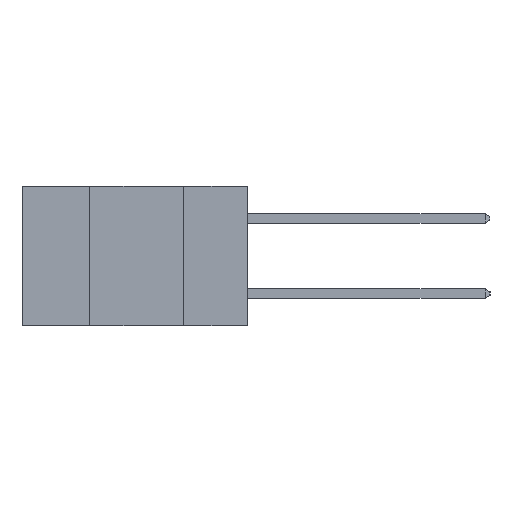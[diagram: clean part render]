
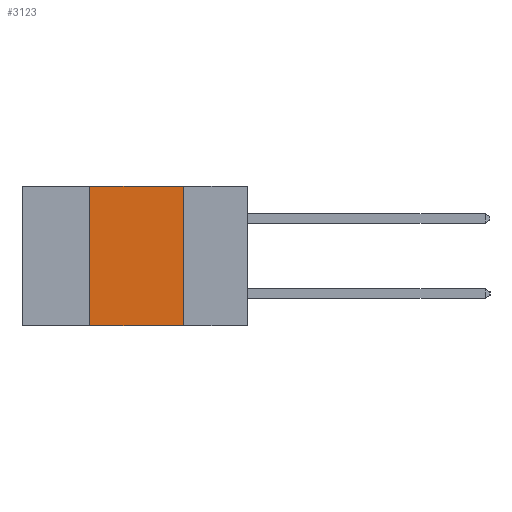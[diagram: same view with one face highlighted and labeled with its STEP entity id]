
A CAD part, left-side view. The second image highlights one B-rep face of the part: STEP entity #3123.
In plain terms, the highlighted planar face has unit normal (-1, 0, 0).
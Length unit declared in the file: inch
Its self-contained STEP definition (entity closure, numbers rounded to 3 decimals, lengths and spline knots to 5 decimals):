
#16 = DIRECTION ( 'NONE',  ( 0., -1., 0. ) ) ;
#35 = CARTESIAN_POINT ( 'NONE',  ( 0., 0.6, 0. ) ) ;
#113 = CARTESIAN_POINT ( 'NONE',  ( 0., 0.42, 0. ) ) ;
#798 = VERTEX_POINT ( 'NONE', #6234 ) ;
#1554 = LINE ( 'NONE', #13496, #13535 ) ;
#2076 = VECTOR ( 'NONE', #3724, 39.37008 ) ;
#3123 = ADVANCED_FACE ( 'NONE', ( #10093 ), #5273, .F. ) ;
#3167 = VERTEX_POINT ( 'NONE', #113 ) ;
#3724 = DIRECTION ( 'NONE',  ( 0., -1., 0. ) ) ;
#3820 = CARTESIAN_POINT ( 'NONE',  ( 0., 0.6, -0.37 ) ) ;
#5273 = PLANE ( 'NONE',  #7773 ) ;
#5826 = LINE ( 'NONE', #35, #14524 ) ;
#6234 = CARTESIAN_POINT ( 'NONE',  ( 0., 0.42, -0.37 ) ) ;
#6297 = VECTOR ( 'NONE', #13851, 39.37008 ) ;
#7108 = VERTEX_POINT ( 'NONE', #8680 ) ;
#7237 = EDGE_CURVE ( 'NONE', #798, #8459, #14017, .T. ) ;
#7324 = ORIENTED_EDGE ( 'NONE', *, *, #7237, .T. ) ;
#7567 = ORIENTED_EDGE ( 'NONE', *, *, #11128, .F. ) ;
#7773 = AXIS2_PLACEMENT_3D ( 'NONE', #12137, #12057, #12977 ) ;
#8005 = EDGE_CURVE ( 'NONE', #798, #3167, #9766, .T. ) ;
#8413 = ORIENTED_EDGE ( 'NONE', *, *, #9570, .F. ) ;
#8459 = VERTEX_POINT ( 'NONE', #10171 ) ;
#8680 = CARTESIAN_POINT ( 'NONE',  ( 0., 0.17, 0. ) ) ;
#9298 = ORIENTED_EDGE ( 'NONE', *, *, #8005, .F. ) ;
#9570 = EDGE_CURVE ( 'NONE', #3167, #7108, #5826, .T. ) ;
#9766 = LINE ( 'NONE', #13958, #6297 ) ;
#10093 = FACE_OUTER_BOUND ( 'NONE', #12132, .T. ) ;
#10171 = CARTESIAN_POINT ( 'NONE',  ( 0., 0.17, -0.37 ) ) ;
#11128 = EDGE_CURVE ( 'NONE', #7108, #8459, #1554, .T. ) ;
#12057 = DIRECTION ( 'NONE',  ( 1., 0., 0. ) ) ;
#12132 = EDGE_LOOP ( 'NONE', ( #7567, #8413, #9298, #7324 ) ) ;
#12137 = CARTESIAN_POINT ( 'NONE',  ( 0., 0.6, 0. ) ) ;
#12977 = DIRECTION ( 'NONE',  ( 0., 0., -1. ) ) ;
#13496 = CARTESIAN_POINT ( 'NONE',  ( 0., 0.17, -0.37 ) ) ;
#13535 = VECTOR ( 'NONE', #13648, 39.37008 ) ;
#13648 = DIRECTION ( 'NONE',  ( 0., 0., -1. ) ) ;
#13851 = DIRECTION ( 'NONE',  ( 0., 0., 1. ) ) ;
#13958 = CARTESIAN_POINT ( 'NONE',  ( 0., 0.42, -0.37 ) ) ;
#14017 = LINE ( 'NONE', #3820, #2076 ) ;
#14524 = VECTOR ( 'NONE', #16, 39.37008 ) ;
